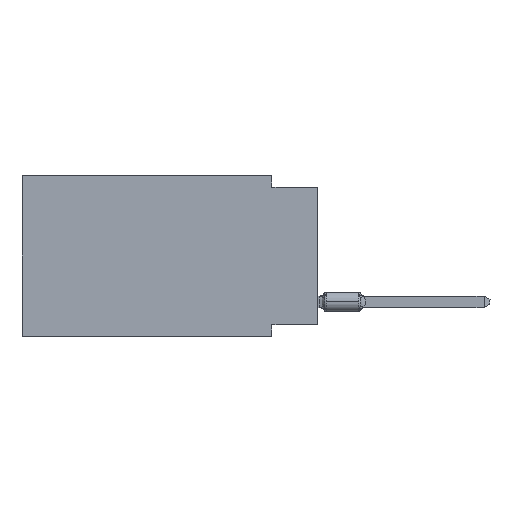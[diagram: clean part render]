
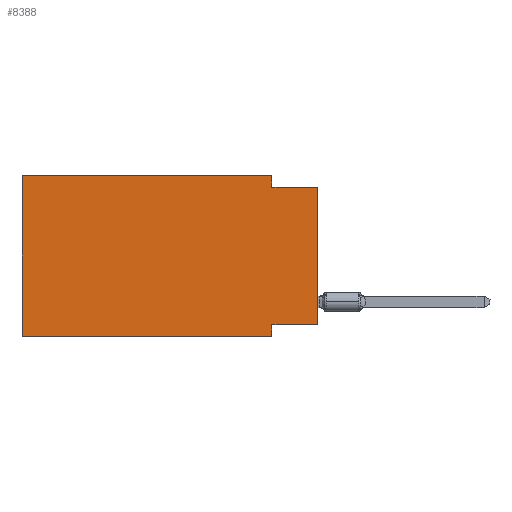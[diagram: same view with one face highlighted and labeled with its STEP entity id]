
A CAD part, left-side view. The second image highlights one B-rep face of the part: STEP entity #8388.
In plain terms, the highlighted planar face has unit normal (-1, 0, 0).
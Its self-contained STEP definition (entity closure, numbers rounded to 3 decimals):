
#914 = DIRECTION ( 'NONE',  ( 0., 0., -1. ) ) ;
#1211 = CARTESIAN_POINT ( 'NONE',  ( 0., 0., 0. ) ) ;
#1322 = EDGE_CURVE ( 'NONE', #1673, #14823, #19362, .T. ) ;
#1642 = CARTESIAN_POINT ( 'NONE',  ( 0., 16.383, -8.89 ) ) ;
#1673 = VERTEX_POINT ( 'NONE', #1988 ) ;
#1729 = DIRECTION ( 'NONE',  ( 0., -1., 0. ) ) ;
#1868 = CARTESIAN_POINT ( 'NONE',  ( 0., 16.383, 0. ) ) ;
#1988 = CARTESIAN_POINT ( 'NONE',  ( 0., 16.383, 0. ) ) ;
#2007 = LINE ( 'NONE', #9921, #29529 ) ;
#2716 = CARTESIAN_POINT ( 'NONE',  ( 0., 2.54, 0. ) ) ;
#2768 = DIRECTION ( 'NONE',  ( 0., 0., 1. ) ) ;
#3390 = LINE ( 'NONE', #3555, #4410 ) ;
#3555 = CARTESIAN_POINT ( 'NONE',  ( 0., 2.54, 0. ) ) ;
#3910 = ORIENTED_EDGE ( 'NONE', *, *, #24297, .T. ) ;
#4410 = VECTOR ( 'NONE', #30300, 1000. ) ;
#4730 = VECTOR ( 'NONE', #11384, 1000. ) ;
#5346 = CARTESIAN_POINT ( 'NONE',  ( 0., 16.383, 0. ) ) ;
#5405 = VECTOR ( 'NONE', #914, 1000. ) ;
#5987 = LINE ( 'NONE', #1211, #4730 ) ;
#6002 = CARTESIAN_POINT ( 'NONE',  ( 0., 2.54, -8.89 ) ) ;
#6086 = EDGE_CURVE ( 'NONE', #25512, #16079, #9344, .T. ) ;
#7077 = VECTOR ( 'NONE', #1729, 1000. ) ;
#7292 = VECTOR ( 'NONE', #16497, 1000. ) ;
#7984 = VERTEX_POINT ( 'NONE', #12701 ) ;
#8336 = CARTESIAN_POINT ( 'NONE',  ( 0., 0., -8.255 ) ) ;
#8388 = ADVANCED_FACE ( 'NONE', ( #15219 ), #12664, .F. ) ;
#9344 = LINE ( 'NONE', #21301, #7077 ) ;
#9921 = CARTESIAN_POINT ( 'NONE',  ( 0., 16.383, 0. ) ) ;
#11157 = EDGE_CURVE ( 'NONE', #7984, #1673, #2007, .T. ) ;
#11384 = DIRECTION ( 'NONE',  ( 0., 0., 1. ) ) ;
#11567 = ORIENTED_EDGE ( 'NONE', *, *, #29386, .F. ) ;
#12664 = PLANE ( 'NONE',  #29276 ) ;
#12701 = CARTESIAN_POINT ( 'NONE',  ( 0., 16.383, -8.89 ) ) ;
#13413 = LINE ( 'NONE', #1642, #25598 ) ;
#14242 = VERTEX_POINT ( 'NONE', #22845 ) ;
#14823 = VERTEX_POINT ( 'NONE', #2716 ) ;
#15219 = FACE_OUTER_BOUND ( 'NONE', #16753, .T. ) ;
#15368 = DIRECTION ( 'NONE',  ( 1., 0., 0. ) ) ;
#15425 = CARTESIAN_POINT ( 'NONE',  ( 0., 2.54, -0.635 ) ) ;
#16079 = VERTEX_POINT ( 'NONE', #20327 ) ;
#16335 = ORIENTED_EDGE ( 'NONE', *, *, #21549, .T. ) ;
#16497 = DIRECTION ( 'NONE',  ( 0., -1., 0. ) ) ;
#16753 = EDGE_LOOP ( 'NONE', ( #3910, #23187, #11567, #23223, #27210, #16335, #19821, #24538 ) ) ;
#16911 = EDGE_CURVE ( 'NONE', #21132, #14242, #22720, .T. ) ;
#18074 = DIRECTION ( 'NONE',  ( 0., 0., -1. ) ) ;
#19362 = LINE ( 'NONE', #1868, #7292 ) ;
#19821 = ORIENTED_EDGE ( 'NONE', *, *, #16911, .F. ) ;
#20018 = CARTESIAN_POINT ( 'NONE',  ( 0., 0., -8.255 ) ) ;
#20327 = CARTESIAN_POINT ( 'NONE',  ( 0., 0., -0.635 ) ) ;
#21132 = VERTEX_POINT ( 'NONE', #29544 ) ;
#21301 = CARTESIAN_POINT ( 'NONE',  ( 0., 0., -0.635 ) ) ;
#21549 = EDGE_CURVE ( 'NONE', #7984, #14242, #13413, .T. ) ;
#22633 = VECTOR ( 'NONE', #30327, 1000. ) ;
#22720 = LINE ( 'NONE', #6002, #5405 ) ;
#22845 = CARTESIAN_POINT ( 'NONE',  ( 0., 2.54, -8.89 ) ) ;
#23187 = ORIENTED_EDGE ( 'NONE', *, *, #6086, .F. ) ;
#23223 = ORIENTED_EDGE ( 'NONE', *, *, #1322, .F. ) ;
#24297 = EDGE_CURVE ( 'NONE', #30312, #16079, #5987, .T. ) ;
#24538 = ORIENTED_EDGE ( 'NONE', *, *, #26503, .F. ) ;
#25233 = LINE ( 'NONE', #8336, #22633 ) ;
#25512 = VERTEX_POINT ( 'NONE', #15425 ) ;
#25598 = VECTOR ( 'NONE', #29723, 1000. ) ;
#26503 = EDGE_CURVE ( 'NONE', #30312, #21132, #25233, .T. ) ;
#27210 = ORIENTED_EDGE ( 'NONE', *, *, #11157, .F. ) ;
#29276 = AXIS2_PLACEMENT_3D ( 'NONE', #5346, #15368, #18074 ) ;
#29386 = EDGE_CURVE ( 'NONE', #14823, #25512, #3390, .T. ) ;
#29529 = VECTOR ( 'NONE', #2768, 1000. ) ;
#29544 = CARTESIAN_POINT ( 'NONE',  ( 0., 2.54, -8.255 ) ) ;
#29723 = DIRECTION ( 'NONE',  ( 0., -1., 0. ) ) ;
#30300 = DIRECTION ( 'NONE',  ( 0., 0., -1. ) ) ;
#30312 = VERTEX_POINT ( 'NONE', #20018 ) ;
#30327 = DIRECTION ( 'NONE',  ( 0., 1., 0. ) ) ;
